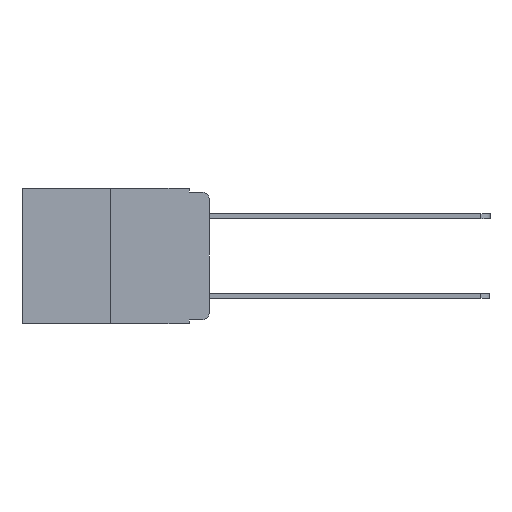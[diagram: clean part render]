
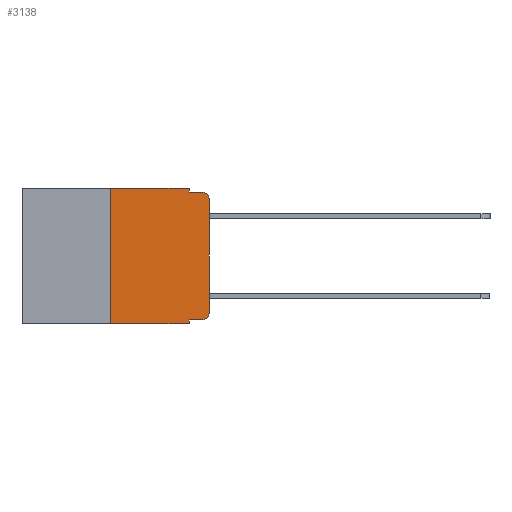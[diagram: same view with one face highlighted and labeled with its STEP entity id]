
A CAD part, left-side view. The second image highlights one B-rep face of the part: STEP entity #3138.
In plain terms, the highlighted planar face has unit normal (-1, 0, 0).
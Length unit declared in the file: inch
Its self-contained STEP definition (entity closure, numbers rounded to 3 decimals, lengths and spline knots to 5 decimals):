
#20 = EDGE_CURVE ( 'NONE', #12907, #11725, #19211, .T. ) ;
#129 = CARTESIAN_POINT ( 'NONE',  ( 0., 0.051, -0.333 ) ) ;
#387 = VERTEX_POINT ( 'NONE', #10462 ) ;
#748 = DIRECTION ( 'NONE',  ( 0., 0., -1. ) ) ;
#1149 = ORIENTED_EDGE ( 'NONE', *, *, #4012, .F. ) ;
#1765 = EDGE_LOOP ( 'NONE', ( #18983, #12373, #16191, #1149, #5508, #17467, #14159, #15091, #3758, #8392 ) ) ;
#1769 = EDGE_CURVE ( 'NONE', #13388, #10984, #18496, .T. ) ;
#1885 = EDGE_CURVE ( 'NONE', #10984, #12907, #7849, .T. ) ;
#3138 = ADVANCED_FACE ( 'NONE', ( #12707 ), #18355, .F. ) ;
#3174 = EDGE_CURVE ( 'NONE', #11725, #17689, #15614, .T. ) ;
#3220 = CARTESIAN_POINT ( 'NONE',  ( 0., 0.25, 0. ) ) ;
#3274 = CARTESIAN_POINT ( 'NONE',  ( 0., 0.473, 0. ) ) ;
#3477 = CARTESIAN_POINT ( 'NONE',  ( 0., 0.051, 0. ) ) ;
#3674 = EDGE_CURVE ( 'NONE', #6198, #17689, #15801, .T. ) ;
#3758 = ORIENTED_EDGE ( 'NONE', *, *, #1769, .T. ) ;
#4012 = EDGE_CURVE ( 'NONE', #13372, #6198, #11987, .T. ) ;
#4163 = CARTESIAN_POINT ( 'NONE',  ( 0., 0.051, -0.333 ) ) ;
#4360 = DIRECTION ( 'NONE',  ( 0., 0., -1. ) ) ;
#4551 = AXIS2_PLACEMENT_3D ( 'NONE', #6751, #12806, #13357 ) ;
#4857 = DIRECTION ( 'NONE',  ( 0., -1., 0. ) ) ;
#5508 = ORIENTED_EDGE ( 'NONE', *, *, #8605, .F. ) ;
#5677 = CARTESIAN_POINT ( 'NONE',  ( 0., 0.02, -0.01 ) ) ;
#5828 = LINE ( 'NONE', #3274, #13122 ) ;
#6136 = DIRECTION ( 'NONE',  ( 0., -1., 0. ) ) ;
#6198 = VERTEX_POINT ( 'NONE', #10233 ) ;
#6397 = DIRECTION ( 'NONE',  ( 0., 0., 1. ) ) ;
#6655 = CARTESIAN_POINT ( 'NONE',  ( 0., 0.473, 0. ) ) ;
#6668 = CARTESIAN_POINT ( 'NONE',  ( 0., 0.473, -0.343 ) ) ;
#6751 = CARTESIAN_POINT ( 'NONE',  ( 0., 0.02, -0.313 ) ) ;
#6963 = VERTEX_POINT ( 'NONE', #15346 ) ;
#7098 = CARTESIAN_POINT ( 'NONE',  ( 0., 0.051, 0. ) ) ;
#7492 = DIRECTION ( 'NONE',  ( 0., -1., 0. ) ) ;
#7601 = VECTOR ( 'NONE', #6136, 39.37008 ) ;
#7849 = CIRCLE ( 'NONE', #4551, 0.02 ) ;
#7866 = LINE ( 'NONE', #18611, #18293 ) ;
#8392 = ORIENTED_EDGE ( 'NONE', *, *, #1885, .T. ) ;
#8605 = EDGE_CURVE ( 'NONE', #15058, #13372, #5828, .T. ) ;
#9686 = CARTESIAN_POINT ( 'NONE',  ( 0., 0., 0. ) ) ;
#10233 = CARTESIAN_POINT ( 'NONE',  ( 0., 0.051, -0.01 ) ) ;
#10386 = CARTESIAN_POINT ( 'NONE',  ( 0., 0.051, -0.01 ) ) ;
#10462 = CARTESIAN_POINT ( 'NONE',  ( 0., 0.051, -0.343 ) ) ;
#10984 = VERTEX_POINT ( 'NONE', #16768 ) ;
#11085 = AXIS2_PLACEMENT_3D ( 'NONE', #6655, #19171, #18151 ) ;
#11725 = VERTEX_POINT ( 'NONE', #12462 ) ;
#11987 = LINE ( 'NONE', #7098, #19041 ) ;
#12219 = VECTOR ( 'NONE', #6397, 39.37008 ) ;
#12373 = ORIENTED_EDGE ( 'NONE', *, *, #3174, .T. ) ;
#12462 = CARTESIAN_POINT ( 'NONE',  ( 0., 0., -0.03 ) ) ;
#12567 = EDGE_CURVE ( 'NONE', #6963, #387, #16041, .T. ) ;
#12684 = VECTOR ( 'NONE', #15325, 39.37008 ) ;
#12707 = FACE_OUTER_BOUND ( 'NONE', #1765, .T. ) ;
#12806 = DIRECTION ( 'NONE',  ( -1., 0., 0. ) ) ;
#12907 = VERTEX_POINT ( 'NONE', #14484 ) ;
#12990 = CARTESIAN_POINT ( 'NONE',  ( 0., 0.02, -0.03 ) ) ;
#13122 = VECTOR ( 'NONE', #4857, 39.37008 ) ;
#13207 = EDGE_CURVE ( 'NONE', #6963, #15058, #16456, .T. ) ;
#13357 = DIRECTION ( 'NONE',  ( 0., 0., -1. ) ) ;
#13372 = VERTEX_POINT ( 'NONE', #3477 ) ;
#13388 = VERTEX_POINT ( 'NONE', #129 ) ;
#13930 = AXIS2_PLACEMENT_3D ( 'NONE', #12990, #17680, #17738 ) ;
#14159 = ORIENTED_EDGE ( 'NONE', *, *, #12567, .T. ) ;
#14484 = CARTESIAN_POINT ( 'NONE',  ( 0., 0., -0.313 ) ) ;
#15058 = VERTEX_POINT ( 'NONE', #15520 ) ;
#15089 = VECTOR ( 'NONE', #15262, 39.37008 ) ;
#15091 = ORIENTED_EDGE ( 'NONE', *, *, #16667, .F. ) ;
#15262 = DIRECTION ( 'NONE',  ( 0., 0., 1. ) ) ;
#15325 = DIRECTION ( 'NONE',  ( 0., -1., 0. ) ) ;
#15346 = CARTESIAN_POINT ( 'NONE',  ( 0., 0.25, -0.343 ) ) ;
#15520 = CARTESIAN_POINT ( 'NONE',  ( 0., 0.25, 0. ) ) ;
#15614 = CIRCLE ( 'NONE', #13930, 0.02 ) ;
#15801 = LINE ( 'NONE', #10386, #16259 ) ;
#16041 = LINE ( 'NONE', #6668, #12684 ) ;
#16191 = ORIENTED_EDGE ( 'NONE', *, *, #3674, .F. ) ;
#16259 = VECTOR ( 'NONE', #7492, 39.37008 ) ;
#16456 = LINE ( 'NONE', #3220, #12219 ) ;
#16667 = EDGE_CURVE ( 'NONE', #13388, #387, #7866, .T. ) ;
#16768 = CARTESIAN_POINT ( 'NONE',  ( 0., 0.02, -0.333 ) ) ;
#17467 = ORIENTED_EDGE ( 'NONE', *, *, #13207, .F. ) ;
#17680 = DIRECTION ( 'NONE',  ( -1., 0., 0. ) ) ;
#17689 = VERTEX_POINT ( 'NONE', #5677 ) ;
#17738 = DIRECTION ( 'NONE',  ( 0., 0., -1. ) ) ;
#18151 = DIRECTION ( 'NONE',  ( 0., 0., -1. ) ) ;
#18293 = VECTOR ( 'NONE', #748, 39.37008 ) ;
#18355 = PLANE ( 'NONE',  #11085 ) ;
#18496 = LINE ( 'NONE', #4163, #7601 ) ;
#18611 = CARTESIAN_POINT ( 'NONE',  ( 0., 0.051, 0. ) ) ;
#18983 = ORIENTED_EDGE ( 'NONE', *, *, #20, .T. ) ;
#19041 = VECTOR ( 'NONE', #4360, 39.37008 ) ;
#19171 = DIRECTION ( 'NONE',  ( 1., 0., 0. ) ) ;
#19211 = LINE ( 'NONE', #9686, #15089 ) ;
